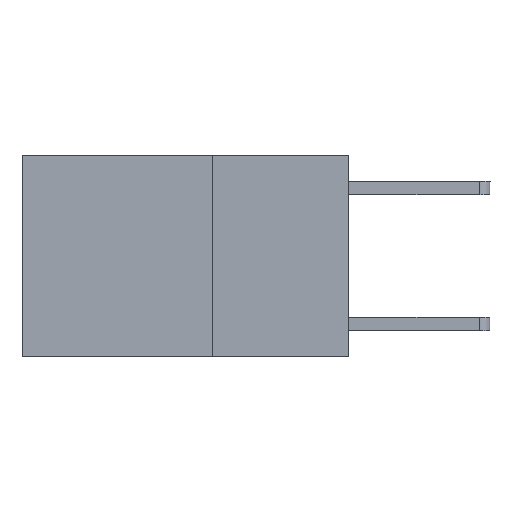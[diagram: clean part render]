
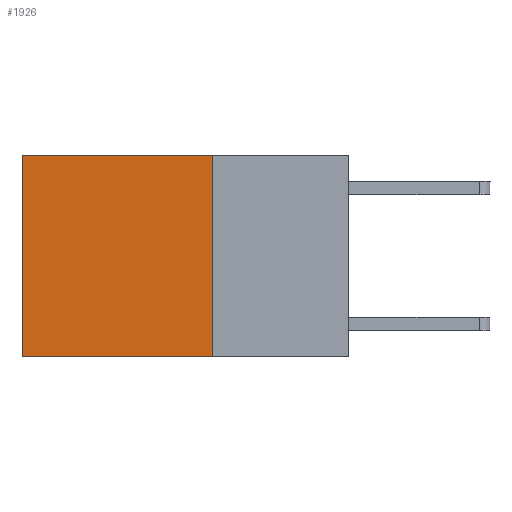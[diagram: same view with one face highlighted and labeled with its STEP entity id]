
A CAD part, left-side view. The second image highlights one B-rep face of the part: STEP entity #1926.
In plain terms, the highlighted planar face has unit normal (-1, 0, 0).
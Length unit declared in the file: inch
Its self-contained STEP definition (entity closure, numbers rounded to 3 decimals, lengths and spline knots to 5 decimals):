
#177 = VECTOR ( 'NONE', #3200, 39.37008 ) ;
#435 = VECTOR ( 'NONE', #4699, 39.37008 ) ;
#574 = CARTESIAN_POINT ( 'NONE',  ( 0.2625, 0.25, -0.37 ) ) ;
#578 = ORIENTED_EDGE ( 'NONE', *, *, #3357, .F. ) ;
#1097 = PLANE ( 'NONE',  #6340 ) ;
#1394 = EDGE_CURVE ( 'NONE', #5963, #6895, #7474, .T. ) ;
#1500 = EDGE_CURVE ( 'NONE', #6895, #5472, #3165, .T. ) ;
#1673 = CARTESIAN_POINT ( 'NONE',  ( 0.2625, 0.25, 0. ) ) ;
#1926 = ADVANCED_FACE ( 'NONE', ( #6838 ), #1097, .F. ) ;
#2413 = DIRECTION ( 'NONE',  ( 0., 0., -1. ) ) ;
#2943 = ORIENTED_EDGE ( 'NONE', *, *, #5029, .F. ) ;
#3089 = VECTOR ( 'NONE', #6214, 39.37008 ) ;
#3165 = LINE ( 'NONE', #5705, #6795 ) ;
#3200 = DIRECTION ( 'NONE',  ( 0., 1., 0. ) ) ;
#3265 = VERTEX_POINT ( 'NONE', #3988 ) ;
#3357 = EDGE_CURVE ( 'NONE', #3265, #5472, #6250, .T. ) ;
#3988 = CARTESIAN_POINT ( 'NONE',  ( 0.2625, 0.25, -0.37 ) ) ;
#4699 = DIRECTION ( 'NONE',  ( 0., 0., -1. ) ) ;
#4741 = ORIENTED_EDGE ( 'NONE', *, *, #1500, .T. ) ;
#5029 = EDGE_CURVE ( 'NONE', #5963, #3265, #6137, .T. ) ;
#5472 = VERTEX_POINT ( 'NONE', #8225 ) ;
#5705 = CARTESIAN_POINT ( 'NONE',  ( 0.2625, 0.6, 0. ) ) ;
#5963 = VERTEX_POINT ( 'NONE', #6482 ) ;
#6039 = CARTESIAN_POINT ( 'NONE',  ( 0.2625, 0.6, 0. ) ) ;
#6137 = LINE ( 'NONE', #1673, #435 ) ;
#6195 = EDGE_LOOP ( 'NONE', ( #4741, #578, #2943, #7307 ) ) ;
#6214 = DIRECTION ( 'NONE',  ( 0., 1., 0. ) ) ;
#6250 = LINE ( 'NONE', #574, #177 ) ;
#6340 = AXIS2_PLACEMENT_3D ( 'NONE', #6437, #7547, #2413 ) ;
#6437 = CARTESIAN_POINT ( 'NONE',  ( 0.2625, 0.25, 0. ) ) ;
#6482 = CARTESIAN_POINT ( 'NONE',  ( 0.2625, 0.25, 0. ) ) ;
#6795 = VECTOR ( 'NONE', #8231, 39.37008 ) ;
#6838 = FACE_OUTER_BOUND ( 'NONE', #6195, .T. ) ;
#6895 = VERTEX_POINT ( 'NONE', #6039 ) ;
#7247 = CARTESIAN_POINT ( 'NONE',  ( 0.2625, 0.25, 0. ) ) ;
#7307 = ORIENTED_EDGE ( 'NONE', *, *, #1394, .T. ) ;
#7474 = LINE ( 'NONE', #7247, #3089 ) ;
#7547 = DIRECTION ( 'NONE',  ( 1., 0., 0. ) ) ;
#8225 = CARTESIAN_POINT ( 'NONE',  ( 0.2625, 0.6, -0.37 ) ) ;
#8231 = DIRECTION ( 'NONE',  ( 0., 0., -1. ) ) ;
